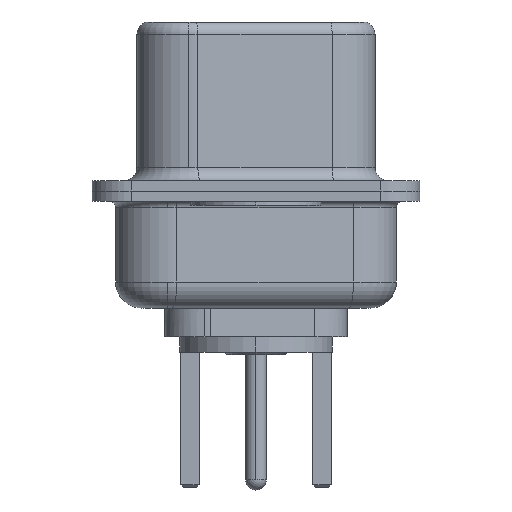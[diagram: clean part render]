
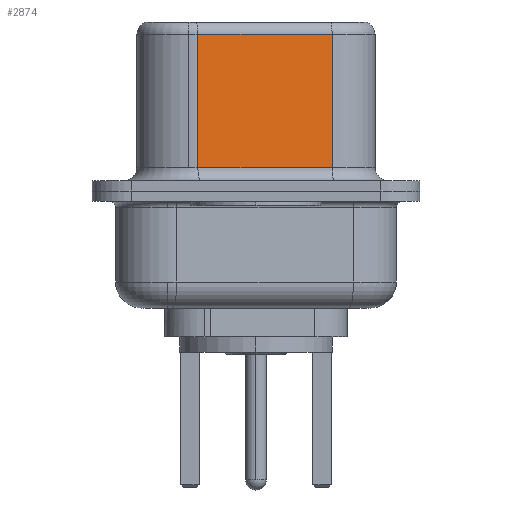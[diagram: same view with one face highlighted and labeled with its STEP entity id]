
A CAD part, left-side view. The second image highlights one B-rep face of the part: STEP entity #2874.
In plain terms, the highlighted planar face has unit normal (-0.985, -0.174, 0).
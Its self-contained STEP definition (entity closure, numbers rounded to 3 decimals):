
#192 = VERTEX_POINT ( 'NONE', #14893 ) ;
#460 = LINE ( 'NONE', #16016, #10161 ) ;
#730 = DIRECTION ( 'NONE',  ( 0., 0., -1. ) ) ;
#1121 = EDGE_CURVE ( 'NONE', #11777, #13584, #460, .T. ) ;
#1358 = ORIENTED_EDGE ( 'NONE', *, *, #15391, .F. ) ;
#2365 = ORIENTED_EDGE ( 'NONE', *, *, #3928, .T. ) ;
#2470 = CARTESIAN_POINT ( 'NONE',  ( 3.67, 2.233, 6.52 ) ) ;
#2874 = ADVANCED_FACE ( 'NONE', ( #3408 ), #11939, .F. ) ;
#3408 = FACE_OUTER_BOUND ( 'NONE', #6911, .T. ) ;
#3886 = CARTESIAN_POINT ( 'NONE',  ( 4.58, -2.927, 6.52 ) ) ;
#3928 = EDGE_CURVE ( 'NONE', #13584, #192, #9142, .T. ) ;
#4450 = DIRECTION ( 'NONE',  ( 0., 0., -1. ) ) ;
#4642 = CARTESIAN_POINT ( 'NONE',  ( 4.58, -2.927, 0.9 ) ) ;
#4980 = CARTESIAN_POINT ( 'NONE',  ( 3.67, 2.233, 6.02 ) ) ;
#5809 = VECTOR ( 'NONE', #4450, 1000. ) ;
#6221 = LINE ( 'NONE', #10830, #12789 ) ;
#6911 = EDGE_LOOP ( 'NONE', ( #1358, #7301, #2365, #8286 ) ) ;
#7301 = ORIENTED_EDGE ( 'NONE', *, *, #1121, .T. ) ;
#8286 = ORIENTED_EDGE ( 'NONE', *, *, #15370, .T. ) ;
#8886 = CARTESIAN_POINT ( 'NONE',  ( 4.58, -2.927, 6.02 ) ) ;
#9142 = LINE ( 'NONE', #2470, #5809 ) ;
#9653 = DIRECTION ( 'NONE',  ( -0.174, 0.985, 0. ) ) ;
#9926 = VECTOR ( 'NONE', #14487, 1000. ) ;
#10161 = VECTOR ( 'NONE', #10201, 1000. ) ;
#10201 = DIRECTION ( 'NONE',  ( -0.174, 0.985, 0. ) ) ;
#10676 = CARTESIAN_POINT ( 'NONE',  ( 4.58, -2.927, 0.9 ) ) ;
#10830 = CARTESIAN_POINT ( 'NONE',  ( 4.58, -2.927, 6.52 ) ) ;
#11777 = VERTEX_POINT ( 'NONE', #8886 ) ;
#11939 = PLANE ( 'NONE',  #15932 ) ;
#12657 = DIRECTION ( 'NONE',  ( 0.985, 0.174, 0. ) ) ;
#12789 = VECTOR ( 'NONE', #730, 1000. ) ;
#13143 = LINE ( 'NONE', #4642, #9926 ) ;
#13358 = VERTEX_POINT ( 'NONE', #10676 ) ;
#13584 = VERTEX_POINT ( 'NONE', #4980 ) ;
#14487 = DIRECTION ( 'NONE',  ( 0.174, -0.985, 0. ) ) ;
#14893 = CARTESIAN_POINT ( 'NONE',  ( 3.67, 2.233, 0.9 ) ) ;
#15370 = EDGE_CURVE ( 'NONE', #192, #13358, #13143, .T. ) ;
#15391 = EDGE_CURVE ( 'NONE', #11777, #13358, #6221, .T. ) ;
#15932 = AXIS2_PLACEMENT_3D ( 'NONE', #3886, #12657, #9653 ) ;
#16016 = CARTESIAN_POINT ( 'NONE',  ( 4.58, -2.927, 6.02 ) ) ;
